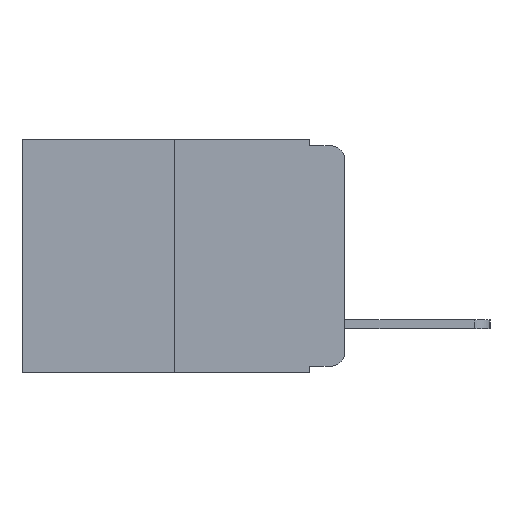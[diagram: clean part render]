
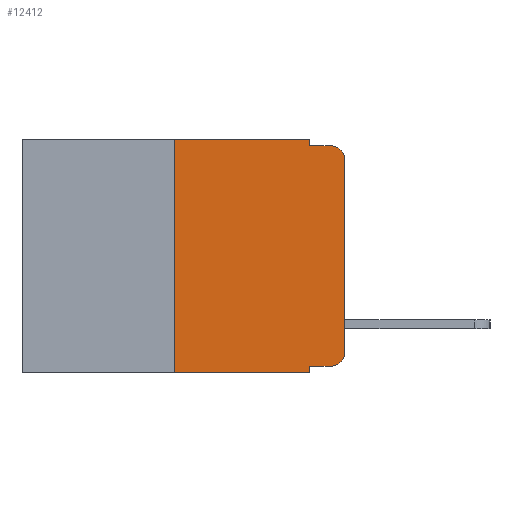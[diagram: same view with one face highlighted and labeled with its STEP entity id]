
A CAD part, left-side view. The second image highlights one B-rep face of the part: STEP entity #12412.
In plain terms, the highlighted planar face has unit normal (-1, 0, 0).
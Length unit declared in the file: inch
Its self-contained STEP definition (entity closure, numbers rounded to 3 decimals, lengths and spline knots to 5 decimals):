
#352 = EDGE_CURVE ( 'NONE', #7866, #9438, #6331, .T. ) ;
#419 = DIRECTION ( 'NONE',  ( 0., 0., -1. ) ) ;
#434 = DIRECTION ( 'NONE',  ( -1., 0., 0. ) ) ;
#551 = CARTESIAN_POINT ( 'NONE',  ( 0., 0.473, 0. ) ) ;
#672 = VERTEX_POINT ( 'NONE', #10658 ) ;
#703 = CARTESIAN_POINT ( 'NONE',  ( 0., 0.02, -0.313 ) ) ;
#792 = EDGE_CURVE ( 'NONE', #4275, #10904, #6695, .T. ) ;
#831 = VECTOR ( 'NONE', #9524, 39.37008 ) ;
#892 = CARTESIAN_POINT ( 'NONE',  ( 0., 0., -0.03 ) ) ;
#1148 = CARTESIAN_POINT ( 'NONE',  ( 0., 0., -0.313 ) ) ;
#1263 = DIRECTION ( 'NONE',  ( -1., 0., 0. ) ) ;
#1399 = VERTEX_POINT ( 'NONE', #12531 ) ;
#1547 = CARTESIAN_POINT ( 'NONE',  ( 0., 0.051, -0.01 ) ) ;
#2217 = CARTESIAN_POINT ( 'NONE',  ( 0., 0.051, -0.333 ) ) ;
#2299 = DIRECTION ( 'NONE',  ( 0., -1., 0. ) ) ;
#2937 = EDGE_LOOP ( 'NONE', ( #11662, #14760, #8801, #12046, #12766, #3388, #9948, #7001, #10332, #4553 ) ) ;
#3214 = LINE ( 'NONE', #10462, #9396 ) ;
#3388 = ORIENTED_EDGE ( 'NONE', *, *, #352, .F. ) ;
#3491 = CARTESIAN_POINT ( 'NONE',  ( 0., 0.473, 0. ) ) ;
#3859 = VERTEX_POINT ( 'NONE', #8147 ) ;
#4092 = CARTESIAN_POINT ( 'NONE',  ( 0., 0.25, 0. ) ) ;
#4275 = VERTEX_POINT ( 'NONE', #15459 ) ;
#4520 = AXIS2_PLACEMENT_3D ( 'NONE', #703, #434, #419 ) ;
#4553 = ORIENTED_EDGE ( 'NONE', *, *, #792, .T. ) ;
#4880 = CARTESIAN_POINT ( 'NONE',  ( 0., 0.051, 0. ) ) ;
#5209 = VECTOR ( 'NONE', #15546, 39.37008 ) ;
#5483 = PLANE ( 'NONE',  #11810 ) ;
#5534 = DIRECTION ( 'NONE',  ( 0., 0., -1. ) ) ;
#5678 = CARTESIAN_POINT ( 'NONE',  ( 0., 0.25, 0. ) ) ;
#5856 = VECTOR ( 'NONE', #2299, 39.37008 ) ;
#6025 = VECTOR ( 'NONE', #11383, 39.37008 ) ;
#6331 = LINE ( 'NONE', #4092, #9666 ) ;
#6402 = CARTESIAN_POINT ( 'NONE',  ( 0., 0.051, 0. ) ) ;
#6492 = EDGE_CURVE ( 'NONE', #12884, #672, #3214, .T. ) ;
#6618 = LINE ( 'NONE', #1547, #6025 ) ;
#6671 = DIRECTION ( 'NONE',  ( 0., -1., 0. ) ) ;
#6686 = DIRECTION ( 'NONE',  ( 1., 0., 0. ) ) ;
#6694 = AXIS2_PLACEMENT_3D ( 'NONE', #8633, #1263, #9860 ) ;
#6695 = CIRCLE ( 'NONE', #4520, 0.02 ) ;
#6857 = CARTESIAN_POINT ( 'NONE',  ( 0., 0.25, -0.343 ) ) ;
#6890 = CARTESIAN_POINT ( 'NONE',  ( 0., 0.051, -0.333 ) ) ;
#7001 = ORIENTED_EDGE ( 'NONE', *, *, #11604, .F. ) ;
#7176 = EDGE_CURVE ( 'NONE', #7866, #3859, #15498, .T. ) ;
#7866 = VERTEX_POINT ( 'NONE', #6857 ) ;
#8147 = CARTESIAN_POINT ( 'NONE',  ( 0., 0.051, -0.343 ) ) ;
#8335 = LINE ( 'NONE', #4880, #14325 ) ;
#8633 = CARTESIAN_POINT ( 'NONE',  ( 0., 0.02, -0.03 ) ) ;
#8801 = ORIENTED_EDGE ( 'NONE', *, *, #15092, .F. ) ;
#9164 = LINE ( 'NONE', #3491, #5856 ) ;
#9396 = VECTOR ( 'NONE', #5534, 39.37008 ) ;
#9438 = VERTEX_POINT ( 'NONE', #5678 ) ;
#9524 = DIRECTION ( 'NONE',  ( 0., 0., 1. ) ) ;
#9581 = EDGE_CURVE ( 'NONE', #9438, #12884, #9164, .T. ) ;
#9666 = VECTOR ( 'NONE', #11057, 39.37008 ) ;
#9860 = DIRECTION ( 'NONE',  ( 0., 0., -1. ) ) ;
#9948 = ORIENTED_EDGE ( 'NONE', *, *, #7176, .T. ) ;
#10332 = ORIENTED_EDGE ( 'NONE', *, *, #12618, .T. ) ;
#10462 = CARTESIAN_POINT ( 'NONE',  ( 0., 0.051, 0. ) ) ;
#10653 = LINE ( 'NONE', #10751, #831 ) ;
#10658 = CARTESIAN_POINT ( 'NONE',  ( 0., 0.051, -0.01 ) ) ;
#10734 = VERTEX_POINT ( 'NONE', #6890 ) ;
#10751 = CARTESIAN_POINT ( 'NONE',  ( 0., 0., 0. ) ) ;
#10904 = VERTEX_POINT ( 'NONE', #1148 ) ;
#10964 = EDGE_CURVE ( 'NONE', #13756, #1399, #14690, .T. ) ;
#11057 = DIRECTION ( 'NONE',  ( 0., 0., 1. ) ) ;
#11383 = DIRECTION ( 'NONE',  ( 0., -1., 0. ) ) ;
#11450 = EDGE_CURVE ( 'NONE', #10904, #13756, #10653, .T. ) ;
#11565 = FACE_OUTER_BOUND ( 'NONE', #2937, .T. ) ;
#11604 = EDGE_CURVE ( 'NONE', #10734, #3859, #8335, .T. ) ;
#11662 = ORIENTED_EDGE ( 'NONE', *, *, #11450, .T. ) ;
#11810 = AXIS2_PLACEMENT_3D ( 'NONE', #551, #6686, #15144 ) ;
#12046 = ORIENTED_EDGE ( 'NONE', *, *, #6492, .F. ) ;
#12113 = LINE ( 'NONE', #2217, #5209 ) ;
#12408 = VECTOR ( 'NONE', #6671, 39.37008 ) ;
#12412 = ADVANCED_FACE ( 'NONE', ( #11565 ), #5483, .F. ) ;
#12531 = CARTESIAN_POINT ( 'NONE',  ( 0., 0.02, -0.01 ) ) ;
#12618 = EDGE_CURVE ( 'NONE', #10734, #4275, #12113, .T. ) ;
#12766 = ORIENTED_EDGE ( 'NONE', *, *, #9581, .F. ) ;
#12884 = VERTEX_POINT ( 'NONE', #6402 ) ;
#13756 = VERTEX_POINT ( 'NONE', #892 ) ;
#14325 = VECTOR ( 'NONE', #15724, 39.37008 ) ;
#14690 = CIRCLE ( 'NONE', #6694, 0.02 ) ;
#14760 = ORIENTED_EDGE ( 'NONE', *, *, #10964, .T. ) ;
#15092 = EDGE_CURVE ( 'NONE', #672, #1399, #6618, .T. ) ;
#15133 = CARTESIAN_POINT ( 'NONE',  ( 0., 0.473, -0.343 ) ) ;
#15144 = DIRECTION ( 'NONE',  ( 0., 0., -1. ) ) ;
#15459 = CARTESIAN_POINT ( 'NONE',  ( 0., 0.02, -0.333 ) ) ;
#15498 = LINE ( 'NONE', #15133, #12408 ) ;
#15546 = DIRECTION ( 'NONE',  ( 0., -1., 0. ) ) ;
#15724 = DIRECTION ( 'NONE',  ( 0., 0., -1. ) ) ;
